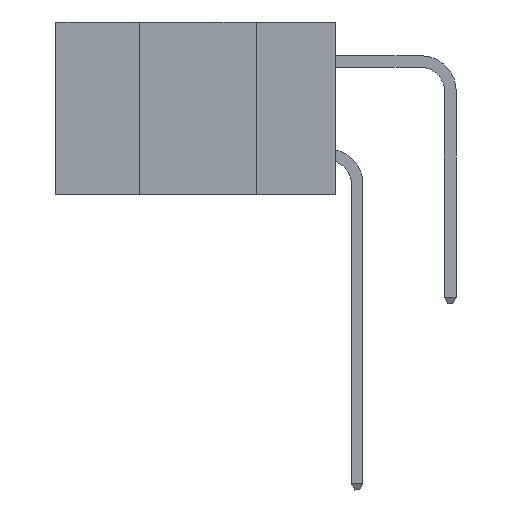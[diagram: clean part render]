
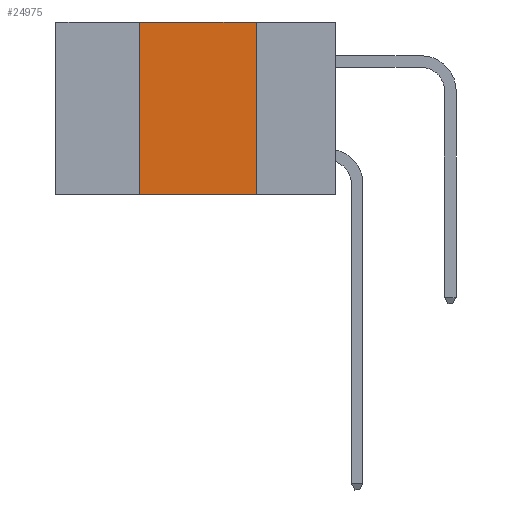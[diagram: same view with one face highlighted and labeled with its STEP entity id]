
A CAD part, left-side view. The second image highlights one B-rep face of the part: STEP entity #24975.
In plain terms, the highlighted planar face has unit normal (-1, 0, 0).
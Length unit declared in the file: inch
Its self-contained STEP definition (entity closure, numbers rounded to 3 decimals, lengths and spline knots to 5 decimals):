
#56 = FACE_OUTER_BOUND ( 'NONE', #27118, .T. ) ;
#533 = VERTEX_POINT ( 'NONE', #34279 ) ;
#1499 = ORIENTED_EDGE ( 'NONE', *, *, #33455, .F. ) ;
#3411 = CARTESIAN_POINT ( 'NONE',  ( 0., 0.17, -0.37 ) ) ;
#7288 = EDGE_CURVE ( 'NONE', #27055, #31924, #27132, .T. ) ;
#8081 = CARTESIAN_POINT ( 'NONE',  ( 0., 0.42, 0. ) ) ;
#9023 = VECTOR ( 'NONE', #20157, 39.37008 ) ;
#11388 = PLANE ( 'NONE',  #21137 ) ;
#11647 = VECTOR ( 'NONE', #32838, 39.37008 ) ;
#11785 = DIRECTION ( 'NONE',  ( 0., 0., -1. ) ) ;
#19530 = CARTESIAN_POINT ( 'NONE',  ( 0., 0.6, 0. ) ) ;
#19606 = CARTESIAN_POINT ( 'NONE',  ( 0., 0.42, -0.37 ) ) ;
#19716 = ORIENTED_EDGE ( 'NONE', *, *, #20834, .F. ) ;
#20157 = DIRECTION ( 'NONE',  ( 0., 0., 1. ) ) ;
#20792 = CARTESIAN_POINT ( 'NONE',  ( 0., 0.6, -0.37 ) ) ;
#20834 = EDGE_CURVE ( 'NONE', #27055, #533, #29654, .T. ) ;
#21137 = AXIS2_PLACEMENT_3D ( 'NONE', #23436, #24219, #11785 ) ;
#23436 = CARTESIAN_POINT ( 'NONE',  ( 0., 0.6, 0. ) ) ;
#23979 = DIRECTION ( 'NONE',  ( 0., 0., -1. ) ) ;
#24161 = LINE ( 'NONE', #32858, #26330 ) ;
#24219 = DIRECTION ( 'NONE',  ( 1., 0., 0. ) ) ;
#24670 = VERTEX_POINT ( 'NONE', #28213 ) ;
#24975 = ADVANCED_FACE ( 'NONE', ( #56 ), #11388, .F. ) ;
#26330 = VECTOR ( 'NONE', #23979, 39.37008 ) ;
#27055 = VERTEX_POINT ( 'NONE', #19606 ) ;
#27060 = VECTOR ( 'NONE', #28615, 39.37008 ) ;
#27118 = EDGE_LOOP ( 'NONE', ( #1499, #34401, #19716, #36696 ) ) ;
#27132 = LINE ( 'NONE', #20792, #11647 ) ;
#28213 = CARTESIAN_POINT ( 'NONE',  ( 0., 0.17, 0. ) ) ;
#28492 = EDGE_CURVE ( 'NONE', #533, #24670, #34535, .T. ) ;
#28615 = DIRECTION ( 'NONE',  ( 0., -1., 0. ) ) ;
#29654 = LINE ( 'NONE', #8081, #9023 ) ;
#31924 = VERTEX_POINT ( 'NONE', #3411 ) ;
#32838 = DIRECTION ( 'NONE',  ( 0., -1., 0. ) ) ;
#32858 = CARTESIAN_POINT ( 'NONE',  ( 0., 0.17, 0. ) ) ;
#33455 = EDGE_CURVE ( 'NONE', #24670, #31924, #24161, .T. ) ;
#34279 = CARTESIAN_POINT ( 'NONE',  ( 0., 0.42, 0. ) ) ;
#34401 = ORIENTED_EDGE ( 'NONE', *, *, #28492, .F. ) ;
#34535 = LINE ( 'NONE', #19530, #27060 ) ;
#36696 = ORIENTED_EDGE ( 'NONE', *, *, #7288, .T. ) ;
